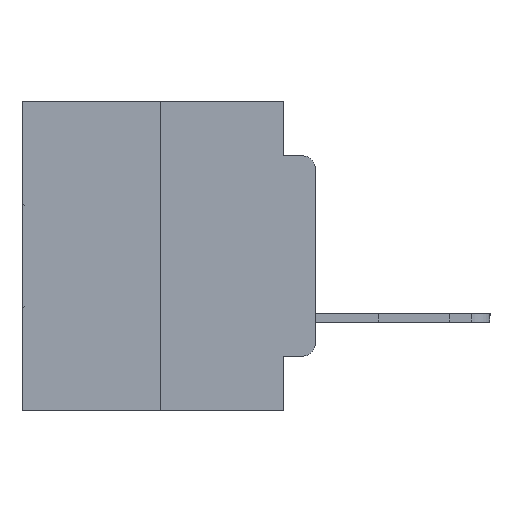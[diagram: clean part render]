
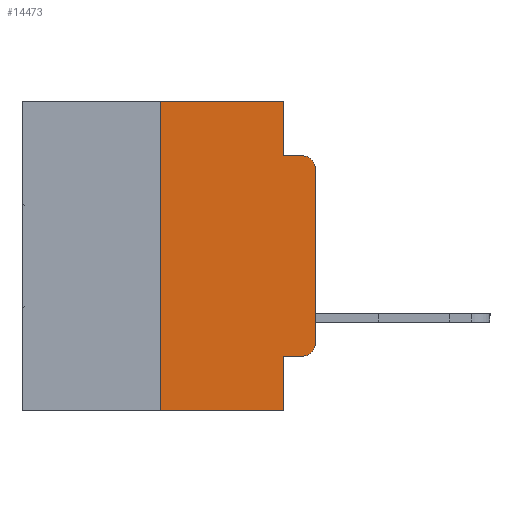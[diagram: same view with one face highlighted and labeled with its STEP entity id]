
A CAD part, left-side view. The second image highlights one B-rep face of the part: STEP entity #14473.
In plain terms, the highlighted planar face has unit normal (-1, 0, 0).
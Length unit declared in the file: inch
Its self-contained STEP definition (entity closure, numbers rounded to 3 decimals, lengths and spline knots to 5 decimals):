
#308 = DIRECTION ( 'NONE',  ( 0., -1., 0. ) ) ;
#598 = CIRCLE ( 'NONE', #15795, 0.02 ) ;
#639 = DIRECTION ( 'NONE',  ( 0., 0., -1. ) ) ;
#1020 = CARTESIAN_POINT ( 'NONE',  ( 0., 0.051, -0.0885 ) ) ;
#1324 = VERTEX_POINT ( 'NONE', #22546 ) ;
#1522 = EDGE_CURVE ( 'NONE', #16390, #20211, #29590, .T. ) ;
#3092 = LINE ( 'NONE', #26730, #7948 ) ;
#3538 = VECTOR ( 'NONE', #10947, 39.37008 ) ;
#3721 = EDGE_CURVE ( 'NONE', #24319, #16390, #12994, .T. ) ;
#3957 = EDGE_CURVE ( 'NONE', #24319, #25408, #11173, .T. ) ;
#4266 = LINE ( 'NONE', #6134, #3538 ) ;
#4336 = CARTESIAN_POINT ( 'NONE',  ( 0., 0.02, -0.1085 ) ) ;
#4832 = VECTOR ( 'NONE', #24793, 39.37008 ) ;
#4999 = EDGE_LOOP ( 'NONE', ( #23456, #5725, #13478, #20891, #21639, #10968, #29322, #30051, #12409, #24588 ) ) ;
#5048 = CARTESIAN_POINT ( 'NONE',  ( 0., 0.02, -0.0885 ) ) ;
#5725 = ORIENTED_EDGE ( 'NONE', *, *, #10116, .T. ) ;
#5845 = DIRECTION ( 'NONE',  ( 0., 0., 1. ) ) ;
#6134 = CARTESIAN_POINT ( 'NONE',  ( 0., 0.051, 0. ) ) ;
#6142 = LINE ( 'NONE', #7710, #30086 ) ;
#6357 = CARTESIAN_POINT ( 'NONE',  ( 0., 0., -0.1085 ) ) ;
#6734 = DIRECTION ( 'NONE',  ( 0., 0., -1. ) ) ;
#6890 = EDGE_CURVE ( 'NONE', #20211, #16283, #4266, .T. ) ;
#7209 = DIRECTION ( 'NONE',  ( 0., -1., 0. ) ) ;
#7430 = CIRCLE ( 'NONE', #25517, 0.02 ) ;
#7710 = CARTESIAN_POINT ( 'NONE',  ( 0., 0.051, 0. ) ) ;
#7874 = CARTESIAN_POINT ( 'NONE',  ( 0., 0.25, 0. ) ) ;
#7898 = VERTEX_POINT ( 'NONE', #5048 ) ;
#7948 = VECTOR ( 'NONE', #5845, 39.37008 ) ;
#8533 = EDGE_CURVE ( 'NONE', #16283, #7898, #16233, .T. ) ;
#10116 = EDGE_CURVE ( 'NONE', #24904, #7898, #7430, .T. ) ;
#10267 = VERTEX_POINT ( 'NONE', #21125 ) ;
#10947 = DIRECTION ( 'NONE',  ( 0., 0., -1. ) ) ;
#10968 = ORIENTED_EDGE ( 'NONE', *, *, #3721, .F. ) ;
#11083 = VECTOR ( 'NONE', #29633, 39.37008 ) ;
#11173 = LINE ( 'NONE', #22439, #4832 ) ;
#11222 = CARTESIAN_POINT ( 'NONE',  ( 0., 0.051, -0.4115 ) ) ;
#11880 = DIRECTION ( 'NONE',  ( -1., 0., 0. ) ) ;
#11916 = CARTESIAN_POINT ( 'NONE',  ( 0., 0.051, 0. ) ) ;
#12409 = ORIENTED_EDGE ( 'NONE', *, *, #26066, .T. ) ;
#12566 = PLANE ( 'NONE',  #25036 ) ;
#12994 = LINE ( 'NONE', #7874, #18299 ) ;
#13478 = ORIENTED_EDGE ( 'NONE', *, *, #8533, .F. ) ;
#14288 = VERTEX_POINT ( 'NONE', #20971 ) ;
#14473 = ADVANCED_FACE ( 'NONE', ( #22939 ), #12566, .F. ) ;
#14828 = DIRECTION ( 'NONE',  ( 0., 0., -1. ) ) ;
#14848 = DIRECTION ( 'NONE',  ( 1., 0., 0. ) ) ;
#15532 = VECTOR ( 'NONE', #308, 39.37008 ) ;
#15795 = AXIS2_PLACEMENT_3D ( 'NONE', #25600, #11880, #27945 ) ;
#16233 = LINE ( 'NONE', #25984, #15532 ) ;
#16283 = VERTEX_POINT ( 'NONE', #1020 ) ;
#16390 = VERTEX_POINT ( 'NONE', #17861 ) ;
#17861 = CARTESIAN_POINT ( 'NONE',  ( 0., 0.25, 0. ) ) ;
#18299 = VECTOR ( 'NONE', #21628, 39.37008 ) ;
#18711 = CARTESIAN_POINT ( 'NONE',  ( 0., 0.473, 0. ) ) ;
#19267 = EDGE_CURVE ( 'NONE', #10267, #24904, #3092, .T. ) ;
#20211 = VERTEX_POINT ( 'NONE', #11916 ) ;
#20532 = DIRECTION ( 'NONE',  ( -1., 0., 0. ) ) ;
#20891 = ORIENTED_EDGE ( 'NONE', *, *, #6890, .F. ) ;
#20971 = CARTESIAN_POINT ( 'NONE',  ( 0., 0.02, -0.4115 ) ) ;
#21125 = CARTESIAN_POINT ( 'NONE',  ( 0., 0., -0.3915 ) ) ;
#21593 = CARTESIAN_POINT ( 'NONE',  ( 0., 0.473, 0. ) ) ;
#21628 = DIRECTION ( 'NONE',  ( 0., 0., 1. ) ) ;
#21639 = ORIENTED_EDGE ( 'NONE', *, *, #1522, .F. ) ;
#21982 = CARTESIAN_POINT ( 'NONE',  ( 0., 0.051, -0.5 ) ) ;
#22439 = CARTESIAN_POINT ( 'NONE',  ( 0., 0.473, -0.5 ) ) ;
#22546 = CARTESIAN_POINT ( 'NONE',  ( 0., 0.051, -0.4115 ) ) ;
#22939 = FACE_OUTER_BOUND ( 'NONE', #4999, .T. ) ;
#23219 = LINE ( 'NONE', #11222, #11083 ) ;
#23456 = ORIENTED_EDGE ( 'NONE', *, *, #19267, .T. ) ;
#24319 = VERTEX_POINT ( 'NONE', #29490 ) ;
#24514 = EDGE_CURVE ( 'NONE', #14288, #10267, #598, .T. ) ;
#24588 = ORIENTED_EDGE ( 'NONE', *, *, #24514, .T. ) ;
#24793 = DIRECTION ( 'NONE',  ( 0., -1., 0. ) ) ;
#24904 = VERTEX_POINT ( 'NONE', #6357 ) ;
#25036 = AXIS2_PLACEMENT_3D ( 'NONE', #21593, #14848, #639 ) ;
#25408 = VERTEX_POINT ( 'NONE', #21982 ) ;
#25517 = AXIS2_PLACEMENT_3D ( 'NONE', #4336, #20532, #6734 ) ;
#25600 = CARTESIAN_POINT ( 'NONE',  ( 0., 0.02, -0.3915 ) ) ;
#25984 = CARTESIAN_POINT ( 'NONE',  ( 0., 0.051, -0.0885 ) ) ;
#26066 = EDGE_CURVE ( 'NONE', #1324, #14288, #23219, .T. ) ;
#26730 = CARTESIAN_POINT ( 'NONE',  ( 0., 0., 0. ) ) ;
#27399 = VECTOR ( 'NONE', #7209, 39.37008 ) ;
#27644 = EDGE_CURVE ( 'NONE', #1324, #25408, #6142, .T. ) ;
#27945 = DIRECTION ( 'NONE',  ( 0., 0., -1. ) ) ;
#29322 = ORIENTED_EDGE ( 'NONE', *, *, #3957, .T. ) ;
#29490 = CARTESIAN_POINT ( 'NONE',  ( 0., 0.25, -0.5 ) ) ;
#29590 = LINE ( 'NONE', #18711, #27399 ) ;
#29633 = DIRECTION ( 'NONE',  ( 0., -1., 0. ) ) ;
#30051 = ORIENTED_EDGE ( 'NONE', *, *, #27644, .F. ) ;
#30086 = VECTOR ( 'NONE', #14828, 39.37008 ) ;
